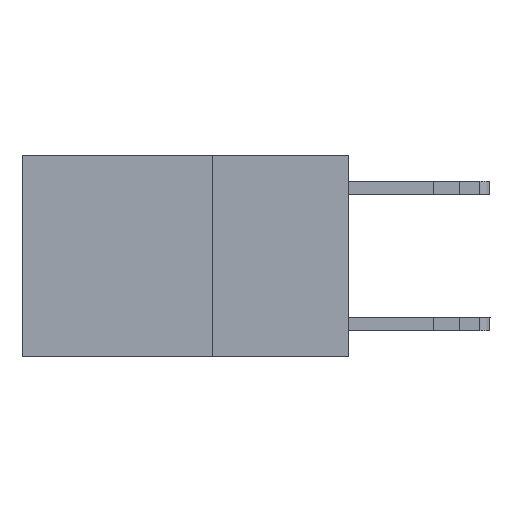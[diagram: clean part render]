
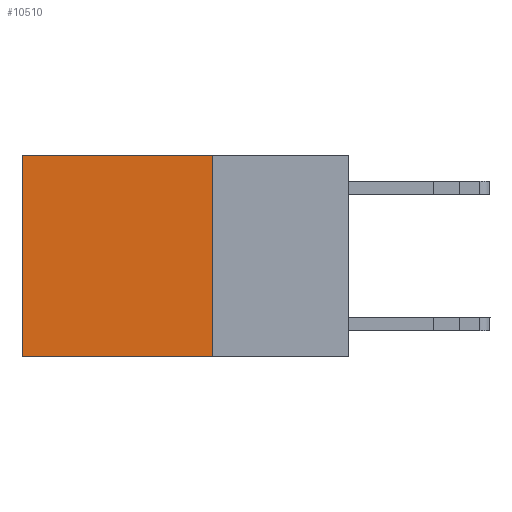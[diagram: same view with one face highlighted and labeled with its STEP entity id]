
A CAD part, left-side view. The second image highlights one B-rep face of the part: STEP entity #10510.
In plain terms, the highlighted planar face has unit normal (-1, 0, 0).
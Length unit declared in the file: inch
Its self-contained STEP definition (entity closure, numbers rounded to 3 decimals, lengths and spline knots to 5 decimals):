
#1343 = PLANE ( 'NONE',  #9090 ) ;
#1405 = DIRECTION ( 'NONE',  ( 0., 0., -1. ) ) ;
#2041 = ORIENTED_EDGE ( 'NONE', *, *, #16135, .T. ) ;
#3091 = ORIENTED_EDGE ( 'NONE', *, *, #8798, .F. ) ;
#4084 = VECTOR ( 'NONE', #11636, 39.37008 ) ;
#4612 = ORIENTED_EDGE ( 'NONE', *, *, #6047, .F. ) ;
#4966 = CARTESIAN_POINT ( 'NONE',  ( 0.2625, 0.25, 0. ) ) ;
#5072 = CARTESIAN_POINT ( 'NONE',  ( 0.2625, 0.25, -0.37 ) ) ;
#5187 = VECTOR ( 'NONE', #14307, 39.37008 ) ;
#5456 = EDGE_LOOP ( 'NONE', ( #2041, #3091, #4612, #6385 ) ) ;
#6020 = LINE ( 'NONE', #11677, #5187 ) ;
#6047 = EDGE_CURVE ( 'NONE', #6894, #12862, #14354, .T. ) ;
#6164 = VERTEX_POINT ( 'NONE', #14405 ) ;
#6226 = LINE ( 'NONE', #8260, #11995 ) ;
#6385 = ORIENTED_EDGE ( 'NONE', *, *, #14253, .T. ) ;
#6894 = VERTEX_POINT ( 'NONE', #16985 ) ;
#7365 = VECTOR ( 'NONE', #14176, 39.37008 ) ;
#7594 = LINE ( 'NONE', #15511, #4084 ) ;
#8260 = CARTESIAN_POINT ( 'NONE',  ( 0.2625, 0.25, 0. ) ) ;
#8798 = EDGE_CURVE ( 'NONE', #12862, #6164, #6020, .T. ) ;
#9090 = AXIS2_PLACEMENT_3D ( 'NONE', #14571, #9366, #1405 ) ;
#9366 = DIRECTION ( 'NONE',  ( 1., 0., 0. ) ) ;
#9370 = CARTESIAN_POINT ( 'NONE',  ( 0.2625, 0.6, 0. ) ) ;
#10510 = ADVANCED_FACE ( 'NONE', ( #10957 ), #1343, .F. ) ;
#10957 = FACE_OUTER_BOUND ( 'NONE', #5456, .T. ) ;
#11636 = DIRECTION ( 'NONE',  ( 0., 0., -1. ) ) ;
#11677 = CARTESIAN_POINT ( 'NONE',  ( 0.2625, 0.25, -0.37 ) ) ;
#11995 = VECTOR ( 'NONE', #13569, 39.37008 ) ;
#12352 = VERTEX_POINT ( 'NONE', #9370 ) ;
#12862 = VERTEX_POINT ( 'NONE', #5072 ) ;
#13569 = DIRECTION ( 'NONE',  ( 0., 1., 0. ) ) ;
#14176 = DIRECTION ( 'NONE',  ( 0., 0., -1. ) ) ;
#14253 = EDGE_CURVE ( 'NONE', #6894, #12352, #6226, .T. ) ;
#14307 = DIRECTION ( 'NONE',  ( 0., 1., 0. ) ) ;
#14354 = LINE ( 'NONE', #4966, #7365 ) ;
#14405 = CARTESIAN_POINT ( 'NONE',  ( 0.2625, 0.6, -0.37 ) ) ;
#14571 = CARTESIAN_POINT ( 'NONE',  ( 0.2625, 0.25, 0. ) ) ;
#15511 = CARTESIAN_POINT ( 'NONE',  ( 0.2625, 0.6, 0. ) ) ;
#16135 = EDGE_CURVE ( 'NONE', #12352, #6164, #7594, .T. ) ;
#16985 = CARTESIAN_POINT ( 'NONE',  ( 0.2625, 0.25, 0. ) ) ;
